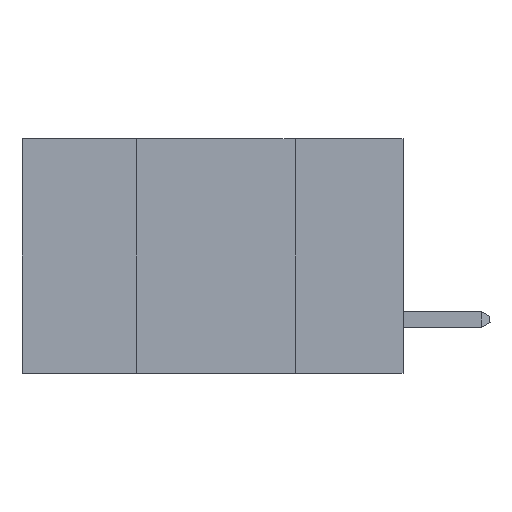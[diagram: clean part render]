
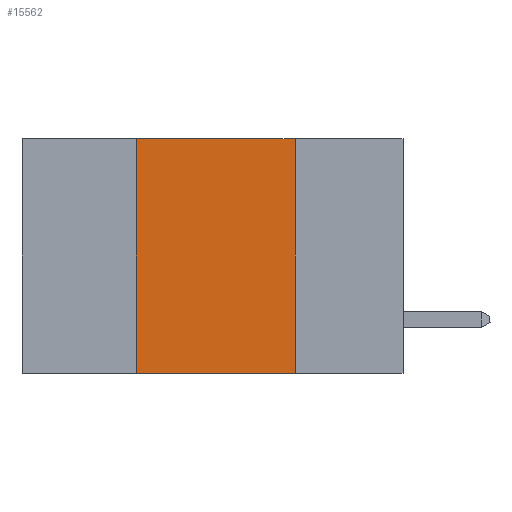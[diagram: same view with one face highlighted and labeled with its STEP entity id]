
A CAD part, left-side view. The second image highlights one B-rep face of the part: STEP entity #15562.
In plain terms, the highlighted planar face has unit normal (-1, 0, 0).
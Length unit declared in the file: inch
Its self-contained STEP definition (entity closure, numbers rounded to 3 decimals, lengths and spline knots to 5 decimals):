
#42 = VECTOR ( 'NONE', #19860, 39.37008 ) ;
#1555 = CARTESIAN_POINT ( 'NONE',  ( 0., 0.17, -0.37 ) ) ;
#4626 = EDGE_CURVE ( 'NONE', #13823, #5816, #8508, .T. ) ;
#5274 = DIRECTION ( 'NONE',  ( 0., 0., -1. ) ) ;
#5816 = VERTEX_POINT ( 'NONE', #6771 ) ;
#6216 = ORIENTED_EDGE ( 'NONE', *, *, #8171, .F. ) ;
#6771 = CARTESIAN_POINT ( 'NONE',  ( 0., 0.42, 0. ) ) ;
#7202 = VERTEX_POINT ( 'NONE', #1555 ) ;
#8171 = EDGE_CURVE ( 'NONE', #5816, #14951, #17638, .T. ) ;
#8233 = ORIENTED_EDGE ( 'NONE', *, *, #8944, .F. ) ;
#8508 = LINE ( 'NONE', #8719, #42 ) ;
#8719 = CARTESIAN_POINT ( 'NONE',  ( 0., 0.42, 0. ) ) ;
#8891 = LINE ( 'NONE', #12004, #9877 ) ;
#8944 = EDGE_CURVE ( 'NONE', #14951, #7202, #16593, .T. ) ;
#9042 = PLANE ( 'NONE',  #17670 ) ;
#9877 = VECTOR ( 'NONE', #13592, 39.37008 ) ;
#10674 = ORIENTED_EDGE ( 'NONE', *, *, #4626, .F. ) ;
#11365 = FACE_OUTER_BOUND ( 'NONE', #19308, .T. ) ;
#12004 = CARTESIAN_POINT ( 'NONE',  ( 0., 0.6, -0.37 ) ) ;
#12126 = DIRECTION ( 'NONE',  ( 1., 0., 0. ) ) ;
#13310 = DIRECTION ( 'NONE',  ( 0., -1., 0. ) ) ;
#13592 = DIRECTION ( 'NONE',  ( 0., -1., 0. ) ) ;
#13823 = VERTEX_POINT ( 'NONE', #17217 ) ;
#14951 = VERTEX_POINT ( 'NONE', #19982 ) ;
#15400 = CARTESIAN_POINT ( 'NONE',  ( 0., 0.6, 0. ) ) ;
#15478 = DIRECTION ( 'NONE',  ( 0., 0., -1. ) ) ;
#15562 = ADVANCED_FACE ( 'NONE', ( #11365 ), #9042, .F. ) ;
#15616 = VECTOR ( 'NONE', #5274, 39.37008 ) ;
#16593 = LINE ( 'NONE', #16655, #15616 ) ;
#16655 = CARTESIAN_POINT ( 'NONE',  ( 0., 0.17, 0. ) ) ;
#17217 = CARTESIAN_POINT ( 'NONE',  ( 0., 0.42, -0.37 ) ) ;
#17638 = LINE ( 'NONE', #18003, #19106 ) ;
#17670 = AXIS2_PLACEMENT_3D ( 'NONE', #15400, #12126, #15478 ) ;
#18003 = CARTESIAN_POINT ( 'NONE',  ( 0., 0.6, 0. ) ) ;
#18043 = ORIENTED_EDGE ( 'NONE', *, *, #20358, .T. ) ;
#19106 = VECTOR ( 'NONE', #13310, 39.37008 ) ;
#19308 = EDGE_LOOP ( 'NONE', ( #8233, #6216, #10674, #18043 ) ) ;
#19860 = DIRECTION ( 'NONE',  ( 0., 0., 1. ) ) ;
#19982 = CARTESIAN_POINT ( 'NONE',  ( 0., 0.17, 0. ) ) ;
#20358 = EDGE_CURVE ( 'NONE', #13823, #7202, #8891, .T. ) ;
